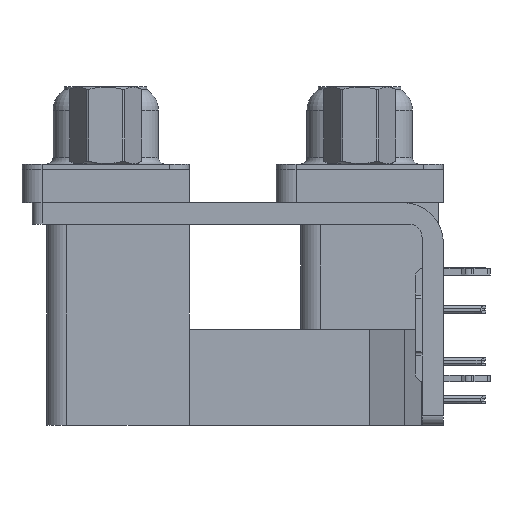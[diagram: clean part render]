
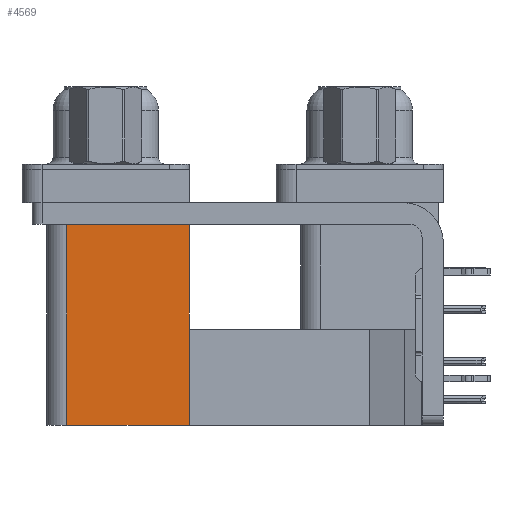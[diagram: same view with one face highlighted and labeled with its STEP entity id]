
A CAD part, left-side view. The second image highlights one B-rep face of the part: STEP entity #4569.
In plain terms, the highlighted planar face has unit normal (-1, 0, 0).
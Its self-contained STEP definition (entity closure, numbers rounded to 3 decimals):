
#2860 = VECTOR ( 'NONE', #24482, 1000. ) ;
#3187 = VERTEX_POINT ( 'NONE', #34536 ) ;
#4215 = LINE ( 'NONE', #19472, #18079 ) ;
#4569 = ADVANCED_FACE ( 'NONE', ( #39798 ), #32250, .F. ) ;
#4596 = VECTOR ( 'NONE', #36382, 1000. ) ;
#5026 = VERTEX_POINT ( 'NONE', #11901 ) ;
#8934 = AXIS2_PLACEMENT_3D ( 'NONE', #13260, #14484, #10248 ) ;
#10248 = DIRECTION ( 'NONE',  ( 0., 1., 0. ) ) ;
#11901 = CARTESIAN_POINT ( 'NONE',  ( 3.79, 12.775, -19.2 ) ) ;
#13260 = CARTESIAN_POINT ( 'NONE',  ( 3.79, 12.775, -19.2 ) ) ;
#14484 = DIRECTION ( 'NONE',  ( 1., 0., 0. ) ) ;
#17815 = EDGE_CURVE ( 'NONE', #3187, #32198, #19629, .T. ) ;
#17847 = CARTESIAN_POINT ( 'NONE',  ( 3.79, 21.975, -19.2 ) ) ;
#18079 = VECTOR ( 'NONE', #23732, 1000. ) ;
#19472 = CARTESIAN_POINT ( 'NONE',  ( 3.79, 12.775, -19.2 ) ) ;
#19629 = LINE ( 'NONE', #35148, #21461 ) ;
#20491 = VERTEX_POINT ( 'NONE', #25901 ) ;
#21461 = VECTOR ( 'NONE', #23885, 1000. ) ;
#23732 = DIRECTION ( 'NONE',  ( 0., 0., 1. ) ) ;
#23885 = DIRECTION ( 'NONE',  ( 0., 1., 0. ) ) ;
#24482 = DIRECTION ( 'NONE',  ( 0., 1., 0. ) ) ;
#24488 = ORIENTED_EDGE ( 'NONE', *, *, #29684, .F. ) ;
#25901 = CARTESIAN_POINT ( 'NONE',  ( 3.79, 21.975, -19.2 ) ) ;
#25963 = EDGE_LOOP ( 'NONE', ( #46218, #24488, #28069, #30679 ) ) ;
#28069 = ORIENTED_EDGE ( 'NONE', *, *, #32064, .F. ) ;
#29684 = EDGE_CURVE ( 'NONE', #20491, #32198, #33109, .T. ) ;
#30679 = ORIENTED_EDGE ( 'NONE', *, *, #30752, .T. ) ;
#30752 = EDGE_CURVE ( 'NONE', #5026, #3187, #4215, .T. ) ;
#32064 = EDGE_CURVE ( 'NONE', #5026, #20491, #35494, .T. ) ;
#32198 = VERTEX_POINT ( 'NONE', #37211 ) ;
#32250 = PLANE ( 'NONE',  #8934 ) ;
#33109 = LINE ( 'NONE', #17847, #4596 ) ;
#34536 = CARTESIAN_POINT ( 'NONE',  ( 3.79, 12.775, -2.5 ) ) ;
#35148 = CARTESIAN_POINT ( 'NONE',  ( 3.79, 12.775, -2.5 ) ) ;
#35494 = LINE ( 'NONE', #39267, #2860 ) ;
#36382 = DIRECTION ( 'NONE',  ( 0., 0., 1. ) ) ;
#37211 = CARTESIAN_POINT ( 'NONE',  ( 3.79, 21.975, -2.5 ) ) ;
#39267 = CARTESIAN_POINT ( 'NONE',  ( 3.79, 12.775, -19.2 ) ) ;
#39798 = FACE_OUTER_BOUND ( 'NONE', #25963, .T. ) ;
#46218 = ORIENTED_EDGE ( 'NONE', *, *, #17815, .T. ) ;
